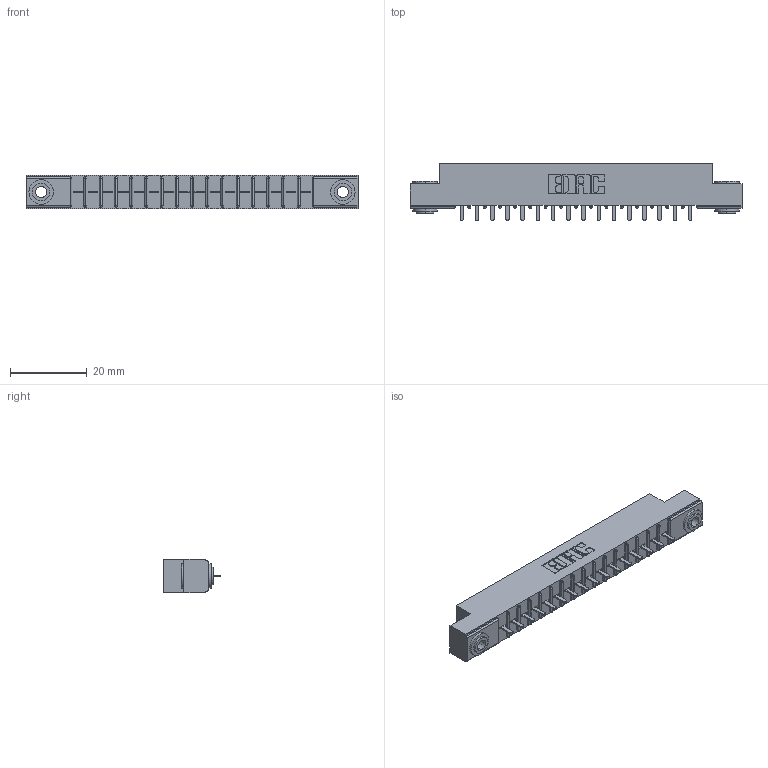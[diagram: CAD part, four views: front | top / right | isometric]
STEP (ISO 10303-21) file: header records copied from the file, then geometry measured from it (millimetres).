
FILE_DESCRIPTION (( 'STEP AP203' ), '1' );
FILE_NAME ('306-016-521-103.STEP', '2019-09-11T20:08:07', ( '' ), ( '' ), 'SwSTEP 2.0', 'SolidWorks 2016', '' );
FILE_SCHEMA (( 'CONFIG_CONTROL_DESIGN' ));
Length unit declared in the file: inch
Products named in the file (4): 306-290-001_121; 306-016-521-103; 345-250-002_345-250-002-102; 306 Part_.156 Dia
Assembly tree (19 placements, depth 2):
  306-016-521-103
    306 Part_.156 Dia
    306-290-001_121  x16
    345-250-002_345-250-002-102  x2
Bounding box: 86.41 x 14.88 x 8.71 mm (x, y, z)
Volume: 5860.1 mm3; surface area: 8625.9 mm2
Topology: 19 solids, 19 shells, 1288 faces, 3580 edges, 2296 vertices
Faces by surface type: plane 844, cylinder 372, sphere 64, cone 8
Entity records: 19310 total; most frequent: CARTESIAN_POINT 3216, DIRECTION 3188, ORIENTED_EDGE 3176, EDGE_CURVE 1588, VECTOR 1220, LINE 1220, VERTEX_POINT 1012, AXIS2_PLACEMENT_3D 984
